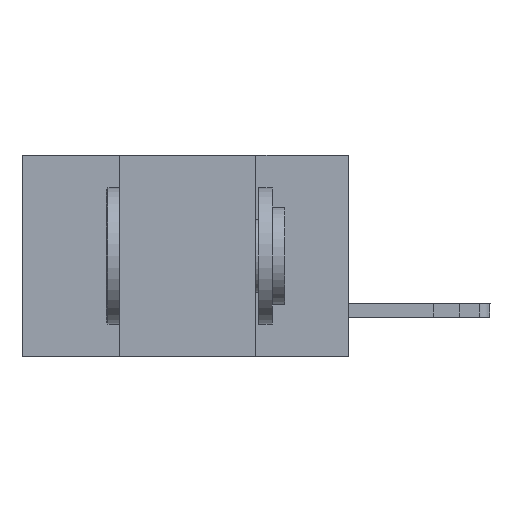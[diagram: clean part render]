
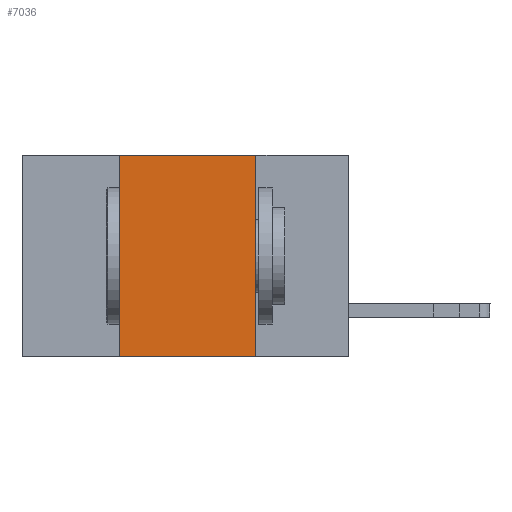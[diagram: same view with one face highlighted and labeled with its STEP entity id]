
A CAD part, left-side view. The second image highlights one B-rep face of the part: STEP entity #7036.
In plain terms, the highlighted planar face has unit normal (-1, 0, 0).
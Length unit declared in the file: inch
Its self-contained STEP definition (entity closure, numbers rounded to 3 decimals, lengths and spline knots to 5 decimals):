
#107 = EDGE_CURVE ( 'NONE', #13846, #285, #9269, .T. ) ;
#285 = VERTEX_POINT ( 'NONE', #10446 ) ;
#905 = VERTEX_POINT ( 'NONE', #6504 ) ;
#1519 = VECTOR ( 'NONE', #16946, 39.37008 ) ;
#1755 = LINE ( 'NONE', #9466, #1519 ) ;
#2155 = CARTESIAN_POINT ( 'NONE',  ( 0., 0.6, -0.37 ) ) ;
#2315 = DIRECTION ( 'NONE',  ( 0., 0., 1. ) ) ;
#2374 = ORIENTED_EDGE ( 'NONE', *, *, #17991, .T. ) ;
#2845 = EDGE_LOOP ( 'NONE', ( #12930, #11837, #7518, #2374 ) ) ;
#3639 = DIRECTION ( 'NONE',  ( 0., -1., 0. ) ) ;
#3856 = EDGE_CURVE ( 'NONE', #905, #13846, #1755, .T. ) ;
#4466 = AXIS2_PLACEMENT_3D ( 'NONE', #10412, #10313, #9199 ) ;
#5510 = VECTOR ( 'NONE', #3639, 39.37008 ) ;
#5947 = FACE_OUTER_BOUND ( 'NONE', #2845, .T. ) ;
#6504 = CARTESIAN_POINT ( 'NONE',  ( 0., 0.42, 0. ) ) ;
#7036 = ADVANCED_FACE ( 'NONE', ( #5947 ), #18087, .F. ) ;
#7518 = ORIENTED_EDGE ( 'NONE', *, *, #15446, .F. ) ;
#9199 = DIRECTION ( 'NONE',  ( 0., 0., -1. ) ) ;
#9269 = LINE ( 'NONE', #16164, #16959 ) ;
#9466 = CARTESIAN_POINT ( 'NONE',  ( 0., 0.6, 0. ) ) ;
#9752 = LINE ( 'NONE', #15626, #11213 ) ;
#10313 = DIRECTION ( 'NONE',  ( 1., 0., 0. ) ) ;
#10412 = CARTESIAN_POINT ( 'NONE',  ( 0., 0.6, 0. ) ) ;
#10446 = CARTESIAN_POINT ( 'NONE',  ( 0., 0.17, -0.37 ) ) ;
#11213 = VECTOR ( 'NONE', #2315, 39.37008 ) ;
#11837 = ORIENTED_EDGE ( 'NONE', *, *, #3856, .F. ) ;
#12880 = LINE ( 'NONE', #2155, #5510 ) ;
#12930 = ORIENTED_EDGE ( 'NONE', *, *, #107, .F. ) ;
#13695 = CARTESIAN_POINT ( 'NONE',  ( 0., 0.17, 0. ) ) ;
#13846 = VERTEX_POINT ( 'NONE', #13695 ) ;
#14571 = CARTESIAN_POINT ( 'NONE',  ( 0., 0.42, -0.37 ) ) ;
#15446 = EDGE_CURVE ( 'NONE', #19325, #905, #9752, .T. ) ;
#15626 = CARTESIAN_POINT ( 'NONE',  ( 0., 0.42, -0.37 ) ) ;
#16164 = CARTESIAN_POINT ( 'NONE',  ( 0., 0.17, -0.37 ) ) ;
#16946 = DIRECTION ( 'NONE',  ( 0., -1., 0. ) ) ;
#16959 = VECTOR ( 'NONE', #19256, 39.37008 ) ;
#17991 = EDGE_CURVE ( 'NONE', #19325, #285, #12880, .T. ) ;
#18087 = PLANE ( 'NONE',  #4466 ) ;
#19256 = DIRECTION ( 'NONE',  ( 0., 0., -1. ) ) ;
#19325 = VERTEX_POINT ( 'NONE', #14571 ) ;
